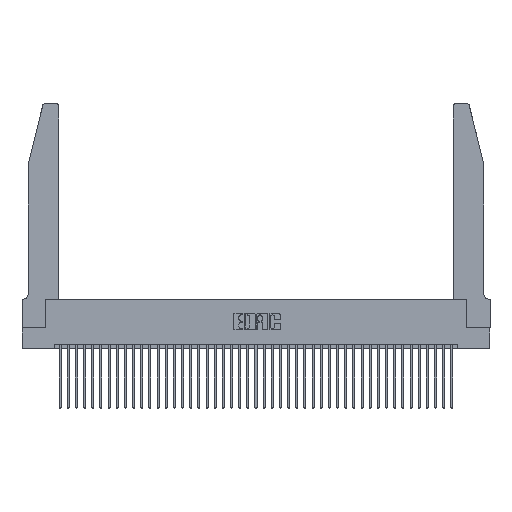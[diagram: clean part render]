
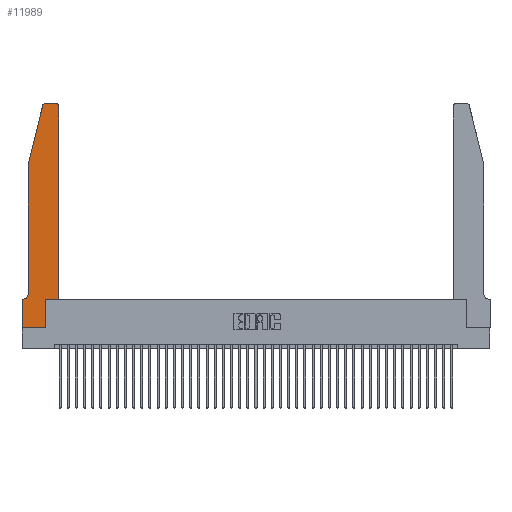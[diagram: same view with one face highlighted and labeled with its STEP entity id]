
A CAD part, top view. The second image highlights one B-rep face of the part: STEP entity #11989.
In plain terms, the highlighted planar face has unit normal (0, 0, 1).
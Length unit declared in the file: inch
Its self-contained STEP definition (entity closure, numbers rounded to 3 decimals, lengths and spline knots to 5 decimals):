
#265 = VERTEX_POINT ( 'NONE', #32662 ) ;
#459 = VERTEX_POINT ( 'NONE', #31637 ) ;
#817 = LINE ( 'NONE', #915, #29031 ) ;
#887 = VECTOR ( 'NONE', #22390, 39.37008 ) ;
#915 = CARTESIAN_POINT ( 'NONE',  ( 0.0755, 0.35, 0.37 ) ) ;
#1012 = DIRECTION ( 'NONE',  ( 1., 0., 0. ) ) ;
#1147 = CARTESIAN_POINT ( 'NONE',  ( 0.4505, 0.35, 0.37 ) ) ;
#1501 = DIRECTION ( 'NONE',  ( -1., 0., 0. ) ) ;
#1635 = CARTESIAN_POINT ( 'NONE',  ( 0.2865, 0., 0.37 ) ) ;
#1638 = ORIENTED_EDGE ( 'NONE', *, *, #31198, .T. ) ;
#3457 = EDGE_CURVE ( 'NONE', #19548, #8339, #6878, .T. ) ;
#4359 = CARTESIAN_POINT ( 'NONE',  ( 0.4505, 2.72, 0.37 ) ) ;
#4633 = ORIENTED_EDGE ( 'NONE', *, *, #6790, .T. ) ;
#4880 = DIRECTION ( 'NONE',  ( 0., 0., 1. ) ) ;
#5591 = DIRECTION ( 'NONE',  ( -1., 0., 0. ) ) ;
#6790 = EDGE_CURVE ( 'NONE', #265, #29902, #20493, .T. ) ;
#6878 = LINE ( 'NONE', #21287, #7900 ) ;
#7754 = DIRECTION ( 'NONE',  ( 1., 0., 0. ) ) ;
#7900 = VECTOR ( 'NONE', #18136, 39.37008 ) ;
#8051 = CARTESIAN_POINT ( 'NONE',  ( 0.0755, 2., 0.37 ) ) ;
#8177 = CARTESIAN_POINT ( 'NONE',  ( 0.25487, 2.72718, 0.37 ) ) ;
#8339 = VERTEX_POINT ( 'NONE', #24494 ) ;
#9322 = EDGE_CURVE ( 'NONE', #19223, #265, #36658, .T. ) ;
#9671 = EDGE_CURVE ( 'NONE', #21134, #39066, #31085, .T. ) ;
#10190 = DIRECTION ( 'NONE',  ( 1., 0., 0. ) ) ;
#10393 = EDGE_CURVE ( 'NONE', #34737, #21134, #41247, .T. ) ;
#10784 = VECTOR ( 'NONE', #11136, 39.37008 ) ;
#10905 = CIRCLE ( 'NONE', #19880, 0.03 ) ;
#11136 = DIRECTION ( 'NONE',  ( 0., 1., 0. ) ) ;
#11457 = CARTESIAN_POINT ( 'NONE',  ( 0., 0.35, 0.37 ) ) ;
#11495 = CARTESIAN_POINT ( 'NONE',  ( 0.4505, 0.35, 0.37 ) ) ;
#11511 = ORIENTED_EDGE ( 'NONE', *, *, #3457, .T. ) ;
#11529 = DIRECTION ( 'NONE',  ( -0.239, -0.971, 0. ) ) ;
#11763 = ORIENTED_EDGE ( 'NONE', *, *, #25585, .T. ) ;
#11989 = ADVANCED_FACE ( 'NONE', ( #12442 ), #24466, .T. ) ;
#12051 = VERTEX_POINT ( 'NONE', #8177 ) ;
#12401 = ORIENTED_EDGE ( 'NONE', *, *, #26026, .T. ) ;
#12442 = FACE_OUTER_BOUND ( 'NONE', #19330, .T. ) ;
#12623 = EDGE_CURVE ( 'NONE', #26652, #34737, #34157, .T. ) ;
#12981 = AXIS2_PLACEMENT_3D ( 'NONE', #23083, #29852, #26395 ) ;
#13134 = ORIENTED_EDGE ( 'NONE', *, *, #9322, .T. ) ;
#14891 = VERTEX_POINT ( 'NONE', #1635 ) ;
#15148 = CARTESIAN_POINT ( 'NONE',  ( 0.2605, 2.75, 0.37 ) ) ;
#16118 = ORIENTED_EDGE ( 'NONE', *, *, #28376, .T. ) ;
#16589 = DIRECTION ( 'NONE',  ( 0., 0., 1. ) ) ;
#17304 = AXIS2_PLACEMENT_3D ( 'NONE', #25797, #25381, #28707 ) ;
#17635 = CARTESIAN_POINT ( 'NONE',  ( 0.4505, 0.35, 0.37 ) ) ;
#18136 = DIRECTION ( 'NONE',  ( 0., -1., 0. ) ) ;
#18688 = ORIENTED_EDGE ( 'NONE', *, *, #28467, .T. ) ;
#19044 = CARTESIAN_POINT ( 'NONE',  ( 0.284, 2.75, 0.37 ) ) ;
#19223 = VERTEX_POINT ( 'NONE', #25523 ) ;
#19224 = CARTESIAN_POINT ( 'NONE',  ( 0., 0., 0.37 ) ) ;
#19330 = EDGE_LOOP ( 'NONE', ( #26679, #16118, #11763, #13134, #4633, #12401, #11511, #36135, #1638, #18688, #20985, #22312 ) ) ;
#19548 = VERTEX_POINT ( 'NONE', #23285 ) ;
#19880 = AXIS2_PLACEMENT_3D ( 'NONE', #23582, #16589, #10190 ) ;
#20493 = CIRCLE ( 'NONE', #17304, 0.07 ) ;
#20654 = AXIS2_PLACEMENT_3D ( 'NONE', #11457, #4880, #7754 ) ;
#20985 = ORIENTED_EDGE ( 'NONE', *, *, #12623, .T. ) ;
#21100 = EDGE_CURVE ( 'NONE', #8339, #14891, #25474, .T. ) ;
#21134 = VERTEX_POINT ( 'NONE', #30096 ) ;
#21287 = CARTESIAN_POINT ( 'NONE',  ( 0., 0., 0.37 ) ) ;
#22312 = ORIENTED_EDGE ( 'NONE', *, *, #10393, .T. ) ;
#22390 = DIRECTION ( 'NONE',  ( 1., 0., 0. ) ) ;
#23083 = CARTESIAN_POINT ( 'NONE',  ( 0.4205, 2.72, 0.37 ) ) ;
#23285 = CARTESIAN_POINT ( 'NONE',  ( 0., 0.35, 0.37 ) ) ;
#23582 = CARTESIAN_POINT ( 'NONE',  ( 0.284, 2.72, 0.37 ) ) ;
#24369 = VECTOR ( 'NONE', #5591, 39.37008 ) ;
#24466 = PLANE ( 'NONE',  #20654 ) ;
#24494 = CARTESIAN_POINT ( 'NONE',  ( 0., 0., 0.37 ) ) ;
#25381 = DIRECTION ( 'NONE',  ( 0., 0., -1. ) ) ;
#25474 = LINE ( 'NONE', #19224, #887 ) ;
#25523 = CARTESIAN_POINT ( 'NONE',  ( 0.0755, 2., 0.37 ) ) ;
#25585 = EDGE_CURVE ( 'NONE', #12051, #19223, #27650, .T. ) ;
#25797 = CARTESIAN_POINT ( 'NONE',  ( 0.0055, 0.42, 0.37 ) ) ;
#26026 = EDGE_CURVE ( 'NONE', #29902, #19548, #817, .T. ) ;
#26395 = DIRECTION ( 'NONE',  ( 1., 0., 0. ) ) ;
#26652 = VERTEX_POINT ( 'NONE', #17635 ) ;
#26679 = ORIENTED_EDGE ( 'NONE', *, *, #9671, .T. ) ;
#27650 = LINE ( 'NONE', #37521, #36299 ) ;
#28376 = EDGE_CURVE ( 'NONE', #39066, #12051, #10905, .T. ) ;
#28467 = EDGE_CURVE ( 'NONE', #459, #26652, #33925, .T. ) ;
#28707 = DIRECTION ( 'NONE',  ( -1., 0., 0. ) ) ;
#28981 = DIRECTION ( 'NONE',  ( 0., 1., 0. ) ) ;
#29031 = VECTOR ( 'NONE', #1501, 39.37008 ) ;
#29852 = DIRECTION ( 'NONE',  ( 0., 0., 1. ) ) ;
#29902 = VERTEX_POINT ( 'NONE', #33496 ) ;
#30096 = CARTESIAN_POINT ( 'NONE',  ( 0.4205, 2.75, 0.37 ) ) ;
#30727 = CARTESIAN_POINT ( 'NONE',  ( 0.2865, 0.35, 0.37 ) ) ;
#31079 = VECTOR ( 'NONE', #40964, 39.37008 ) ;
#31085 = LINE ( 'NONE', #15148, #24369 ) ;
#31198 = EDGE_CURVE ( 'NONE', #14891, #459, #41474, .T. ) ;
#31637 = CARTESIAN_POINT ( 'NONE',  ( 0.2865, 0.35, 0.37 ) ) ;
#32662 = CARTESIAN_POINT ( 'NONE',  ( 0.0755, 0.42, 0.37 ) ) ;
#33496 = CARTESIAN_POINT ( 'NONE',  ( 0.0055, 0.35, 0.37 ) ) ;
#33925 = LINE ( 'NONE', #1147, #40561 ) ;
#34157 = LINE ( 'NONE', #11495, #41837 ) ;
#34737 = VERTEX_POINT ( 'NONE', #4359 ) ;
#36135 = ORIENTED_EDGE ( 'NONE', *, *, #21100, .T. ) ;
#36299 = VECTOR ( 'NONE', #11529, 39.37008 ) ;
#36658 = LINE ( 'NONE', #8051, #31079 ) ;
#37521 = CARTESIAN_POINT ( 'NONE',  ( 0.0755, 2., 0.37 ) ) ;
#39066 = VERTEX_POINT ( 'NONE', #19044 ) ;
#40561 = VECTOR ( 'NONE', #1012, 39.37008 ) ;
#40964 = DIRECTION ( 'NONE',  ( 0., -1., 0. ) ) ;
#41247 = CIRCLE ( 'NONE', #12981, 0.03 ) ;
#41474 = LINE ( 'NONE', #30727, #10784 ) ;
#41837 = VECTOR ( 'NONE', #28981, 39.37008 ) ;
